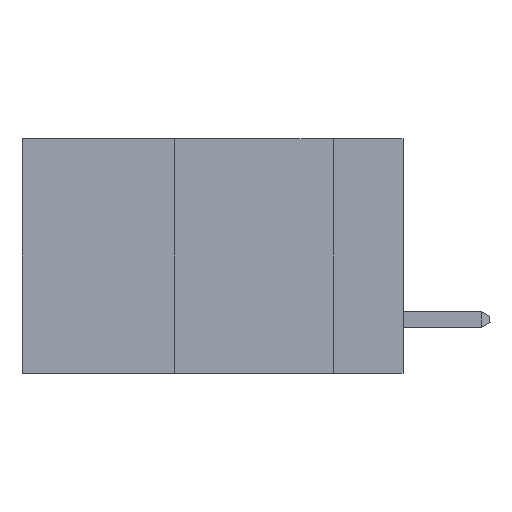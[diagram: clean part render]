
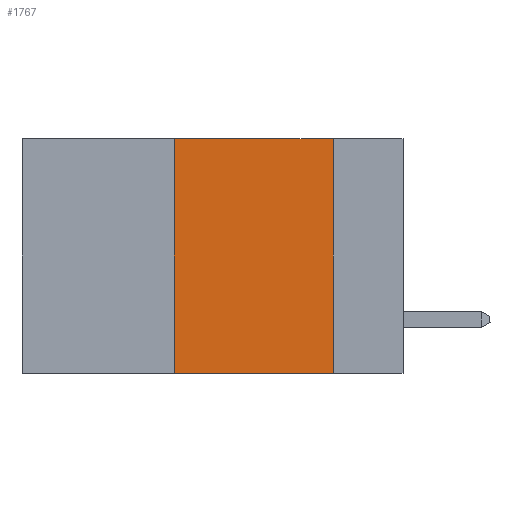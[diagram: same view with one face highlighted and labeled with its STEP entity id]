
A CAD part, left-side view. The second image highlights one B-rep face of the part: STEP entity #1767.
In plain terms, the highlighted planar face has unit normal (-1, 0, 0).
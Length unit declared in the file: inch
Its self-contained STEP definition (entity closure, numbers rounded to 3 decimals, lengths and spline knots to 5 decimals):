
#97 = PLANE ( 'NONE',  #31828 ) ;
#1767 = ADVANCED_FACE ( 'NONE', ( #17966 ), #97, .F. ) ;
#5252 = ORIENTED_EDGE ( 'NONE', *, *, #5864, .T. ) ;
#5864 = EDGE_CURVE ( 'NONE', #31652, #19778, #34516, .T. ) ;
#6274 = CARTESIAN_POINT ( 'NONE',  ( 0., 0.6, 0. ) ) ;
#6277 = CARTESIAN_POINT ( 'NONE',  ( 0., 0.6, 0. ) ) ;
#6609 = DIRECTION ( 'NONE',  ( 0., -1., 0. ) ) ;
#7483 = DIRECTION ( 'NONE',  ( 0., 0., -1. ) ) ;
#7836 = CARTESIAN_POINT ( 'NONE',  ( 0., 0.11, 0. ) ) ;
#8238 = CARTESIAN_POINT ( 'NONE',  ( 0., 0.36, 0. ) ) ;
#8421 = VERTEX_POINT ( 'NONE', #17809 ) ;
#9445 = CARTESIAN_POINT ( 'NONE',  ( 0., 0.6, -0.37 ) ) ;
#10299 = ORIENTED_EDGE ( 'NONE', *, *, #29298, .F. ) ;
#11651 = VECTOR ( 'NONE', #7483, 39.37008 ) ;
#11902 = EDGE_LOOP ( 'NONE', ( #16156, #22465, #10299, #5252 ) ) ;
#13581 = LINE ( 'NONE', #6277, #31779 ) ;
#15455 = EDGE_CURVE ( 'NONE', #8421, #19693, #13581, .T. ) ;
#16156 = ORIENTED_EDGE ( 'NONE', *, *, #23172, .F. ) ;
#16750 = LINE ( 'NONE', #7836, #11651 ) ;
#16988 = CARTESIAN_POINT ( 'NONE',  ( 0., 0.11, 0. ) ) ;
#17192 = VECTOR ( 'NONE', #24710, 39.37008 ) ;
#17809 = CARTESIAN_POINT ( 'NONE',  ( 0., 0.36, 0. ) ) ;
#17966 = FACE_OUTER_BOUND ( 'NONE', #11902, .T. ) ;
#19693 = VERTEX_POINT ( 'NONE', #16988 ) ;
#19778 = VERTEX_POINT ( 'NONE', #25097 ) ;
#22465 = ORIENTED_EDGE ( 'NONE', *, *, #15455, .F. ) ;
#23172 = EDGE_CURVE ( 'NONE', #19693, #19778, #16750, .T. ) ;
#24710 = DIRECTION ( 'NONE',  ( 0., 0., 1. ) ) ;
#24770 = DIRECTION ( 'NONE',  ( 1., 0., 0. ) ) ;
#25097 = CARTESIAN_POINT ( 'NONE',  ( 0., 0.11, -0.37 ) ) ;
#27349 = VECTOR ( 'NONE', #6609, 39.37008 ) ;
#29298 = EDGE_CURVE ( 'NONE', #31652, #8421, #29818, .T. ) ;
#29818 = LINE ( 'NONE', #8238, #17192 ) ;
#30540 = DIRECTION ( 'NONE',  ( 0., 0., -1. ) ) ;
#31652 = VERTEX_POINT ( 'NONE', #31980 ) ;
#31779 = VECTOR ( 'NONE', #33377, 39.37008 ) ;
#31828 = AXIS2_PLACEMENT_3D ( 'NONE', #6274, #24770, #30540 ) ;
#31980 = CARTESIAN_POINT ( 'NONE',  ( 0., 0.36, -0.37 ) ) ;
#33377 = DIRECTION ( 'NONE',  ( 0., -1., 0. ) ) ;
#34516 = LINE ( 'NONE', #9445, #27349 ) ;
